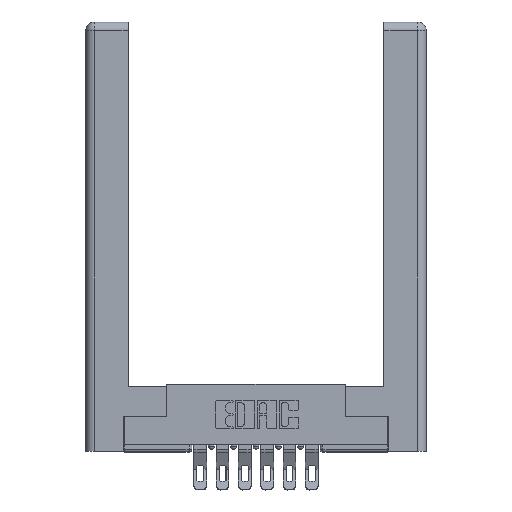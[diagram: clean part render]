
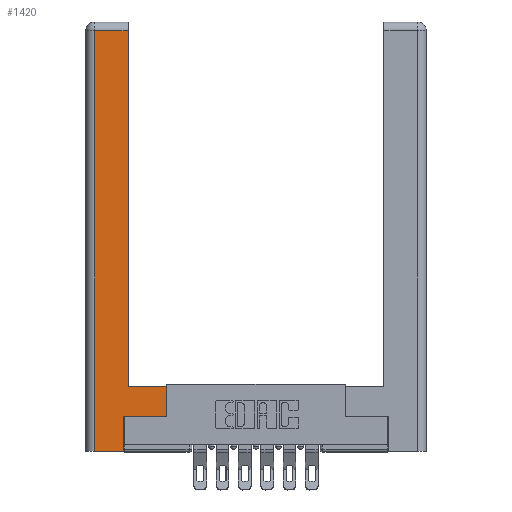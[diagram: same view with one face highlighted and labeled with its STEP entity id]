
A CAD part, top view. The second image highlights one B-rep face of the part: STEP entity #1420.
In plain terms, the highlighted planar face has unit normal (0, 0, 1).
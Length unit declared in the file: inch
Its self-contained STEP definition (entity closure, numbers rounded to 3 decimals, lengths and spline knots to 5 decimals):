
#926 = VERTEX_POINT ( 'NONE', #7927 ) ;
#993 = CARTESIAN_POINT ( 'NONE',  ( 0.265, 0.245, 0. ) ) ;
#1052 = CARTESIAN_POINT ( 'NONE',  ( 0., 0., 0. ) ) ;
#1091 = PLANE ( 'NONE',  #1327 ) ;
#1264 = LINE ( 'NONE', #5593, #5870 ) ;
#1327 = AXIS2_PLACEMENT_3D ( 'NONE', #1052, #8057, #7176 ) ;
#1420 = ADVANCED_FACE ( 'NONE', ( #3821 ), #1091, .F. ) ;
#1455 = VECTOR ( 'NONE', #3501, 39.37008 ) ;
#1664 = VECTOR ( 'NONE', #2892, 39.37008 ) ;
#1890 = DIRECTION ( 'NONE',  ( 0., -1., 0. ) ) ;
#2031 = ORIENTED_EDGE ( 'NONE', *, *, #3626, .T. ) ;
#2081 = VECTOR ( 'NONE', #1890, 39.37008 ) ;
#2356 = VERTEX_POINT ( 'NONE', #4686 ) ;
#2710 = EDGE_CURVE ( 'NONE', #926, #6136, #11829, .T. ) ;
#2877 = LINE ( 'NONE', #5814, #2081 ) ;
#2892 = DIRECTION ( 'NONE',  ( 1., 0., 0. ) ) ;
#3102 = ORIENTED_EDGE ( 'NONE', *, *, #2710, .T. ) ;
#3151 = EDGE_CURVE ( 'NONE', #2356, #7361, #6643, .T. ) ;
#3316 = EDGE_LOOP ( 'NONE', ( #4095, #11052, #3466, #2031, #10218, #8151, #12096, #3102 ) ) ;
#3466 = ORIENTED_EDGE ( 'NONE', *, *, #7665, .T. ) ;
#3501 = DIRECTION ( 'NONE',  ( 0., 1., 0. ) ) ;
#3626 = EDGE_CURVE ( 'NONE', #7464, #2356, #5213, .T. ) ;
#3821 = FACE_OUTER_BOUND ( 'NONE', #3316, .T. ) ;
#3946 = VECTOR ( 'NONE', #4116, 39.37008 ) ;
#4095 = ORIENTED_EDGE ( 'NONE', *, *, #8039, .T. ) ;
#4116 = DIRECTION ( 'NONE',  ( 0., 1., 0. ) ) ;
#4221 = CARTESIAN_POINT ( 'NONE',  ( 0.295, 0.45, 0. ) ) ;
#4686 = CARTESIAN_POINT ( 'NONE',  ( 0.265, 0., 0. ) ) ;
#4949 = DIRECTION ( 'NONE',  ( 0., 1., 0. ) ) ;
#5213 = LINE ( 'NONE', #12591, #6944 ) ;
#5593 = CARTESIAN_POINT ( 'NONE',  ( 0.0615, 2.94, 0. ) ) ;
#5776 = EDGE_CURVE ( 'NONE', #7361, #12622, #7187, .T. ) ;
#5814 = CARTESIAN_POINT ( 'NONE',  ( 0.0615, 0., 0. ) ) ;
#5870 = VECTOR ( 'NONE', #8501, 39.37008 ) ;
#5983 = CARTESIAN_POINT ( 'NONE',  ( 0.565, 0.45, 0. ) ) ;
#6136 = VERTEX_POINT ( 'NONE', #8661 ) ;
#6411 = VERTEX_POINT ( 'NONE', #8052 ) ;
#6425 = CARTESIAN_POINT ( 'NONE',  ( 0.265, 0.245, 0. ) ) ;
#6643 = LINE ( 'NONE', #993, #3946 ) ;
#6944 = VECTOR ( 'NONE', #9888, 39.37008 ) ;
#6967 = VECTOR ( 'NONE', #4949, 39.37008 ) ;
#7042 = CARTESIAN_POINT ( 'NONE',  ( 0.565, 0.245, 0. ) ) ;
#7176 = DIRECTION ( 'NONE',  ( -1., 0., 0. ) ) ;
#7187 = LINE ( 'NONE', #8975, #1664 ) ;
#7189 = DIRECTION ( 'NONE',  ( -1., 0., 0. ) ) ;
#7361 = VERTEX_POINT ( 'NONE', #6425 ) ;
#7464 = VERTEX_POINT ( 'NONE', #11706 ) ;
#7665 = EDGE_CURVE ( 'NONE', #6411, #7464, #2877, .T. ) ;
#7927 = CARTESIAN_POINT ( 'NONE',  ( 0.565, 0.45, 0. ) ) ;
#8039 = EDGE_CURVE ( 'NONE', #6136, #10298, #9021, .T. ) ;
#8052 = CARTESIAN_POINT ( 'NONE',  ( 0.0615, 2.94, 0. ) ) ;
#8057 = DIRECTION ( 'NONE',  ( 0., 0., -1. ) ) ;
#8151 = ORIENTED_EDGE ( 'NONE', *, *, #5776, .T. ) ;
#8501 = DIRECTION ( 'NONE',  ( -1., 0., 0. ) ) ;
#8584 = CARTESIAN_POINT ( 'NONE',  ( 0.295, 2.94, 0. ) ) ;
#8661 = CARTESIAN_POINT ( 'NONE',  ( 0.295, 0.45, 0. ) ) ;
#8860 = VECTOR ( 'NONE', #7189, 39.37008 ) ;
#8975 = CARTESIAN_POINT ( 'NONE',  ( 0.565, 0.245, 0. ) ) ;
#9021 = LINE ( 'NONE', #12379, #1455 ) ;
#9888 = DIRECTION ( 'NONE',  ( 1., 0., 0. ) ) ;
#9958 = EDGE_CURVE ( 'NONE', #12622, #926, #11963, .T. ) ;
#10218 = ORIENTED_EDGE ( 'NONE', *, *, #3151, .T. ) ;
#10298 = VERTEX_POINT ( 'NONE', #8584 ) ;
#10379 = EDGE_CURVE ( 'NONE', #10298, #6411, #1264, .T. ) ;
#11052 = ORIENTED_EDGE ( 'NONE', *, *, #10379, .T. ) ;
#11706 = CARTESIAN_POINT ( 'NONE',  ( 0.0615, 0., 0. ) ) ;
#11829 = LINE ( 'NONE', #4221, #8860 ) ;
#11963 = LINE ( 'NONE', #5983, #6967 ) ;
#12096 = ORIENTED_EDGE ( 'NONE', *, *, #9958, .T. ) ;
#12379 = CARTESIAN_POINT ( 'NONE',  ( 0.295, 3., 0. ) ) ;
#12591 = CARTESIAN_POINT ( 'NONE',  ( 0.265, 0., 0. ) ) ;
#12622 = VERTEX_POINT ( 'NONE', #7042 ) ;
